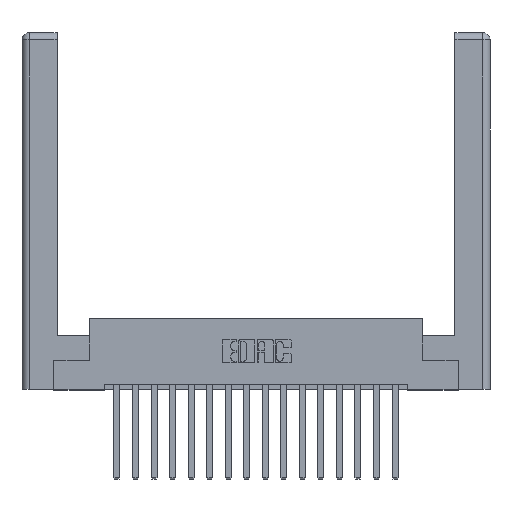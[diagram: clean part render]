
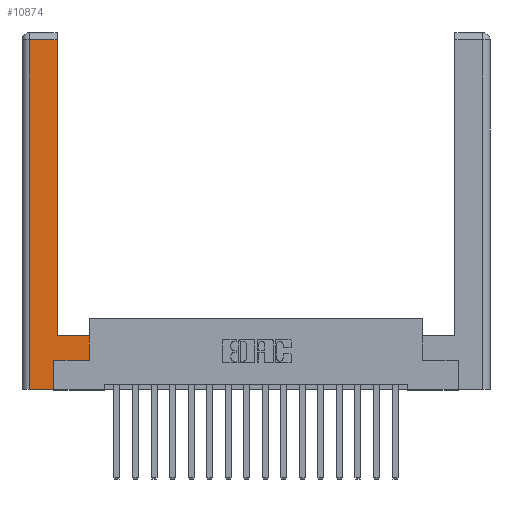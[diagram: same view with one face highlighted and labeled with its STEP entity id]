
A CAD part, top view. The second image highlights one B-rep face of the part: STEP entity #10874.
In plain terms, the highlighted planar face has unit normal (0, 0, 1).
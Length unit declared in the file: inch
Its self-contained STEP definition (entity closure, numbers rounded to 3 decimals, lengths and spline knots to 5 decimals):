
#424 = CARTESIAN_POINT ( 'NONE',  ( 0.0615, 2.94, 0. ) ) ;
#761 = PLANE ( 'NONE',  #7470 ) ;
#1213 = VERTEX_POINT ( 'NONE', #13417 ) ;
#1852 = EDGE_CURVE ( 'NONE', #2347, #1213, #16849, .T. ) ;
#2051 = DIRECTION ( 'NONE',  ( 0., 0., -1. ) ) ;
#2347 = VERTEX_POINT ( 'NONE', #7101 ) ;
#2845 = CARTESIAN_POINT ( 'NONE',  ( 0.265, 0.245, 0. ) ) ;
#3410 = VECTOR ( 'NONE', #12821, 39.37008 ) ;
#3520 = ORIENTED_EDGE ( 'NONE', *, *, #15279, .T. ) ;
#3540 = CARTESIAN_POINT ( 'NONE',  ( 0.265, 0.245, 0. ) ) ;
#3926 = EDGE_CURVE ( 'NONE', #16033, #6758, #14559, .T. ) ;
#4414 = ORIENTED_EDGE ( 'NONE', *, *, #3926, .T. ) ;
#5073 = VECTOR ( 'NONE', #15257, 39.37008 ) ;
#5712 = CARTESIAN_POINT ( 'NONE',  ( 0.565, 0.45, 0. ) ) ;
#5828 = CARTESIAN_POINT ( 'NONE',  ( 0.565, 0.245, 0. ) ) ;
#6050 = EDGE_CURVE ( 'NONE', #1213, #16033, #17885, .T. ) ;
#6055 = ORIENTED_EDGE ( 'NONE', *, *, #12094, .T. ) ;
#6244 = VECTOR ( 'NONE', #13663, 39.37008 ) ;
#6349 = CARTESIAN_POINT ( 'NONE',  ( 0.295, 3., 0. ) ) ;
#6758 = VERTEX_POINT ( 'NONE', #9147 ) ;
#7097 = ORIENTED_EDGE ( 'NONE', *, *, #9451, .T. ) ;
#7101 = CARTESIAN_POINT ( 'NONE',  ( 0.565, 0.245, 0. ) ) ;
#7470 = AXIS2_PLACEMENT_3D ( 'NONE', #9198, #2051, #10681 ) ;
#7568 = CARTESIAN_POINT ( 'NONE',  ( 0.0615, 0., 0. ) ) ;
#7733 = CARTESIAN_POINT ( 'NONE',  ( 0.265, 0., 0. ) ) ;
#9019 = CARTESIAN_POINT ( 'NONE',  ( 0.295, 0.45, 0. ) ) ;
#9031 = VERTEX_POINT ( 'NONE', #7568 ) ;
#9134 = DIRECTION ( 'NONE',  ( 0., 1., 0. ) ) ;
#9147 = CARTESIAN_POINT ( 'NONE',  ( 0.295, 2.94, 0. ) ) ;
#9185 = EDGE_LOOP ( 'NONE', ( #4414, #7097, #6055, #3520, #14447, #12316, #11738, #12489 ) ) ;
#9198 = CARTESIAN_POINT ( 'NONE',  ( 0., 0., 0. ) ) ;
#9205 = DIRECTION ( 'NONE',  ( -1., 0., 0. ) ) ;
#9357 = VERTEX_POINT ( 'NONE', #15240 ) ;
#9451 = EDGE_CURVE ( 'NONE', #6758, #13286, #10685, .T. ) ;
#9822 = LINE ( 'NONE', #7733, #17979 ) ;
#10171 = VECTOR ( 'NONE', #9205, 39.37008 ) ;
#10368 = CARTESIAN_POINT ( 'NONE',  ( 0.0615, 0., 0. ) ) ;
#10394 = CARTESIAN_POINT ( 'NONE',  ( 0.0615, 2.94, 0. ) ) ;
#10524 = DIRECTION ( 'NONE',  ( 1., 0., 0. ) ) ;
#10681 = DIRECTION ( 'NONE',  ( -1., 0., 0. ) ) ;
#10685 = LINE ( 'NONE', #424, #17751 ) ;
#10874 = ADVANCED_FACE ( 'NONE', ( #11038 ), #761, .F. ) ;
#10909 = VERTEX_POINT ( 'NONE', #3540 ) ;
#11038 = FACE_OUTER_BOUND ( 'NONE', #9185, .T. ) ;
#11242 = VECTOR ( 'NONE', #9134, 39.37008 ) ;
#11578 = VECTOR ( 'NONE', #16173, 39.37008 ) ;
#11738 = ORIENTED_EDGE ( 'NONE', *, *, #1852, .T. ) ;
#12094 = EDGE_CURVE ( 'NONE', #13286, #9031, #14684, .T. ) ;
#12316 = ORIENTED_EDGE ( 'NONE', *, *, #13042, .T. ) ;
#12489 = ORIENTED_EDGE ( 'NONE', *, *, #6050, .T. ) ;
#12821 = DIRECTION ( 'NONE',  ( 0., 1., 0. ) ) ;
#13042 = EDGE_CURVE ( 'NONE', #10909, #2347, #14386, .T. ) ;
#13123 = DIRECTION ( 'NONE',  ( -1., 0., 0. ) ) ;
#13286 = VERTEX_POINT ( 'NONE', #10394 ) ;
#13417 = CARTESIAN_POINT ( 'NONE',  ( 0.565, 0.45, 0. ) ) ;
#13663 = DIRECTION ( 'NONE',  ( 1., 0., 0. ) ) ;
#14386 = LINE ( 'NONE', #5828, #6244 ) ;
#14447 = ORIENTED_EDGE ( 'NONE', *, *, #18128, .T. ) ;
#14559 = LINE ( 'NONE', #6349, #11242 ) ;
#14684 = LINE ( 'NONE', #10368, #11578 ) ;
#15240 = CARTESIAN_POINT ( 'NONE',  ( 0.265, 0., 0. ) ) ;
#15257 = DIRECTION ( 'NONE',  ( 0., 1., 0. ) ) ;
#15279 = EDGE_CURVE ( 'NONE', #9031, #9357, #9822, .T. ) ;
#16033 = VERTEX_POINT ( 'NONE', #17906 ) ;
#16173 = DIRECTION ( 'NONE',  ( 0., -1., 0. ) ) ;
#16849 = LINE ( 'NONE', #5712, #3410 ) ;
#17216 = LINE ( 'NONE', #2845, #5073 ) ;
#17751 = VECTOR ( 'NONE', #13123, 39.37008 ) ;
#17885 = LINE ( 'NONE', #9019, #10171 ) ;
#17906 = CARTESIAN_POINT ( 'NONE',  ( 0.295, 0.45, 0. ) ) ;
#17979 = VECTOR ( 'NONE', #10524, 39.37008 ) ;
#18128 = EDGE_CURVE ( 'NONE', #9357, #10909, #17216, .T. ) ;
